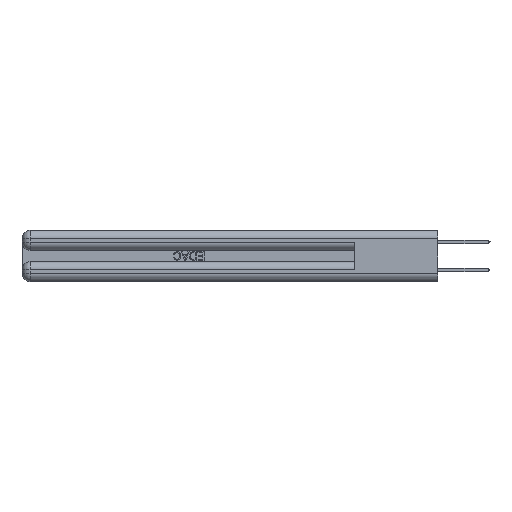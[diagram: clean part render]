
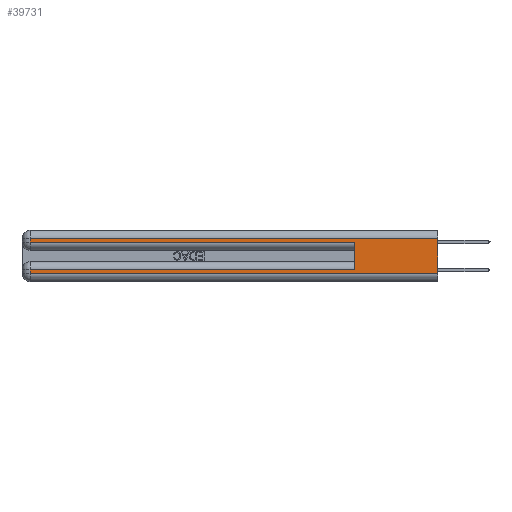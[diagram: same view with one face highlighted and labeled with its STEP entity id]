
A CAD part, left-side view. The second image highlights one B-rep face of the part: STEP entity #39731.
In plain terms, the highlighted planar face has unit normal (-1, 0, 0).
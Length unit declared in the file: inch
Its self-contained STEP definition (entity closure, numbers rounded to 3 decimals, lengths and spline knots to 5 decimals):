
#29 = DIRECTION ( 'NONE',  ( 0., 0., 1. ) ) ;
#1455 = CARTESIAN_POINT ( 'NONE',  ( 0., 2.94, 0.37 ) ) ;
#3122 = DIRECTION ( 'NONE',  ( 0., -1., 0. ) ) ;
#3154 = FACE_OUTER_BOUND ( 'NONE', #34244, .T. ) ;
#3713 = CARTESIAN_POINT ( 'NONE',  ( 0., 0.6, 0.145 ) ) ;
#4407 = LINE ( 'NONE', #19476, #44289 ) ;
#5077 = CARTESIAN_POINT ( 'NONE',  ( 0., 0., 0.37 ) ) ;
#5196 = VECTOR ( 'NONE', #19309, 39.37008 ) ;
#5335 = DIRECTION ( 'NONE',  ( 0., 0., -1. ) ) ;
#6978 = VERTEX_POINT ( 'NONE', #11658 ) ;
#7641 = LINE ( 'NONE', #49805, #5196 ) ;
#7996 = EDGE_CURVE ( 'NONE', #38574, #45606, #39123, .T. ) ;
#8292 = LINE ( 'NONE', #15716, #27739 ) ;
#8994 = DIRECTION ( 'NONE',  ( 0., 0., -1. ) ) ;
#9010 = EDGE_CURVE ( 'NONE', #30663, #20478, #7641, .T. ) ;
#9013 = LINE ( 'NONE', #41650, #27240 ) ;
#9572 = ORIENTED_EDGE ( 'NONE', *, *, #48903, .T. ) ;
#10045 = DIRECTION ( 'NONE',  ( 0., 1., 0. ) ) ;
#11658 = CARTESIAN_POINT ( 'NONE',  ( 0., 0., 0.06 ) ) ;
#13404 = EDGE_CURVE ( 'NONE', #35301, #6978, #9013, .T. ) ;
#14168 = DIRECTION ( 'NONE',  ( 0., 0., -1. ) ) ;
#15716 = CARTESIAN_POINT ( 'NONE',  ( 0., 0., 0.085 ) ) ;
#15743 = ORIENTED_EDGE ( 'NONE', *, *, #16654, .F. ) ;
#16654 = EDGE_CURVE ( 'NONE', #18053, #20478, #34599, .T. ) ;
#17745 = CARTESIAN_POINT ( 'NONE',  ( 0., 0., 0.31 ) ) ;
#18053 = VERTEX_POINT ( 'NONE', #40119 ) ;
#19309 = DIRECTION ( 'NONE',  ( 0., -1., 0. ) ) ;
#19476 = CARTESIAN_POINT ( 'NONE',  ( 0., 0., 0.37 ) ) ;
#19573 = DIRECTION ( 'NONE',  ( 0., 1., 0. ) ) ;
#20478 = VERTEX_POINT ( 'NONE', #49416 ) ;
#21787 = CARTESIAN_POINT ( 'NONE',  ( 0., 2.94, 0.37 ) ) ;
#22062 = EDGE_CURVE ( 'NONE', #38958, #35301, #47644, .T. ) ;
#22354 = CARTESIAN_POINT ( 'NONE',  ( 0., 0., 0.31 ) ) ;
#23845 = CARTESIAN_POINT ( 'NONE',  ( 0., 2.94, 0.085 ) ) ;
#24100 = ORIENTED_EDGE ( 'NONE', *, *, #13404, .T. ) ;
#24362 = VECTOR ( 'NONE', #29, 39.37008 ) ;
#25387 = VECTOR ( 'NONE', #5335, 39.37008 ) ;
#26908 = ORIENTED_EDGE ( 'NONE', *, *, #7996, .T. ) ;
#27240 = VECTOR ( 'NONE', #3122, 39.37008 ) ;
#27480 = EDGE_CURVE ( 'NONE', #18053, #38958, #8292, .T. ) ;
#27739 = VECTOR ( 'NONE', #19573, 39.37008 ) ;
#28364 = PLANE ( 'NONE',  #49880 ) ;
#30179 = ORIENTED_EDGE ( 'NONE', *, *, #36757, .F. ) ;
#30663 = VERTEX_POINT ( 'NONE', #31190 ) ;
#31126 = DIRECTION ( 'NONE',  ( 0., 0., -1. ) ) ;
#31190 = CARTESIAN_POINT ( 'NONE',  ( 0., 2.94, 0.285 ) ) ;
#32200 = DIRECTION ( 'NONE',  ( 1., 0., 0. ) ) ;
#32922 = CARTESIAN_POINT ( 'NONE',  ( 0., 2.94, 0.06 ) ) ;
#34244 = EDGE_LOOP ( 'NONE', ( #30179, #26908, #9572, #37821, #15743, #46174, #41929, #24100 ) ) ;
#34403 = LINE ( 'NONE', #1455, #25387 ) ;
#34599 = LINE ( 'NONE', #3713, #24362 ) ;
#35301 = VERTEX_POINT ( 'NONE', #32922 ) ;
#36757 = EDGE_CURVE ( 'NONE', #38574, #6978, #4407, .T. ) ;
#37550 = VECTOR ( 'NONE', #14168, 39.37008 ) ;
#37821 = ORIENTED_EDGE ( 'NONE', *, *, #9010, .T. ) ;
#38574 = VERTEX_POINT ( 'NONE', #22354 ) ;
#38958 = VERTEX_POINT ( 'NONE', #23845 ) ;
#39123 = LINE ( 'NONE', #17745, #46835 ) ;
#39731 = ADVANCED_FACE ( 'NONE', ( #3154 ), #28364, .F. ) ;
#40119 = CARTESIAN_POINT ( 'NONE',  ( 0., 0.6, 0.085 ) ) ;
#41650 = CARTESIAN_POINT ( 'NONE',  ( 0., 0., 0.06 ) ) ;
#41929 = ORIENTED_EDGE ( 'NONE', *, *, #22062, .T. ) ;
#44289 = VECTOR ( 'NONE', #31126, 39.37008 ) ;
#45606 = VERTEX_POINT ( 'NONE', #48952 ) ;
#46174 = ORIENTED_EDGE ( 'NONE', *, *, #27480, .T. ) ;
#46835 = VECTOR ( 'NONE', #10045, 39.37008 ) ;
#47644 = LINE ( 'NONE', #21787, #37550 ) ;
#48903 = EDGE_CURVE ( 'NONE', #45606, #30663, #34403, .T. ) ;
#48952 = CARTESIAN_POINT ( 'NONE',  ( 0., 2.94, 0.31 ) ) ;
#49416 = CARTESIAN_POINT ( 'NONE',  ( 0., 0.6, 0.285 ) ) ;
#49805 = CARTESIAN_POINT ( 'NONE',  ( 0., 0., 0.285 ) ) ;
#49880 = AXIS2_PLACEMENT_3D ( 'NONE', #5077, #32200, #8994 ) ;
